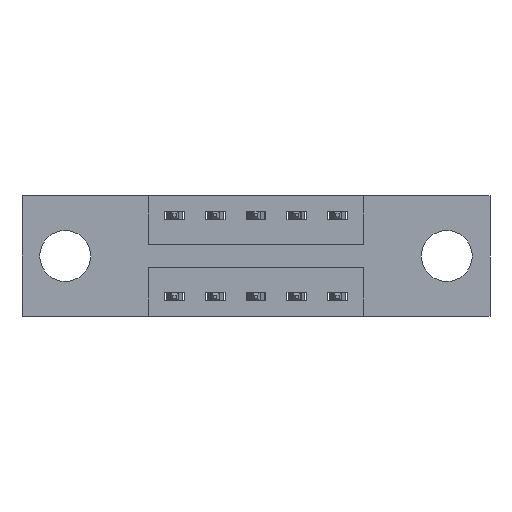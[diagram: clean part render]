
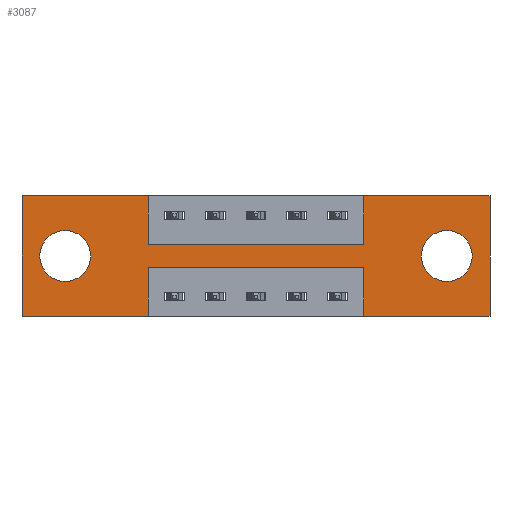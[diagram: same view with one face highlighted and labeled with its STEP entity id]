
A CAD part, front view. The second image highlights one B-rep face of the part: STEP entity #3087.
In plain terms, the highlighted planar face has unit normal (0, -1, 0).
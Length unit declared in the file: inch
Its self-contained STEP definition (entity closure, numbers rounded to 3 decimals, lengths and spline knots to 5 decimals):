
#97 = CARTESIAN_POINT ( 'NONE',  ( 0.3875, 0., -0.15 ) ) ;
#135 = CARTESIAN_POINT ( 'NONE',  ( 1.435, 0., 0. ) ) ;
#159 = ORIENTED_EDGE ( 'NONE', *, *, #3614, .F. ) ;
#218 = CARTESIAN_POINT ( 'NONE',  ( 0., 0., -0.37 ) ) ;
#339 = DIRECTION ( 'NONE',  ( 0., 0., 1. ) ) ;
#363 = ORIENTED_EDGE ( 'NONE', *, *, #2648, .F. ) ;
#393 = FACE_BOUND ( 'NONE', #5636, .T. ) ;
#713 = VERTEX_POINT ( 'NONE', #7406 ) ;
#732 = ORIENTED_EDGE ( 'NONE', *, *, #6379, .F. ) ;
#763 = CARTESIAN_POINT ( 'NONE',  ( 0., 0., -0.37 ) ) ;
#812 = EDGE_CURVE ( 'NONE', #1909, #713, #1612, .T. ) ;
#863 = CARTESIAN_POINT ( 'NONE',  ( 1.0475, 0., -0.37 ) ) ;
#921 = FACE_OUTER_BOUND ( 'NONE', #5794, .T. ) ;
#931 = EDGE_CURVE ( 'NONE', #5371, #4724, #8557, .T. ) ;
#1012 = CARTESIAN_POINT ( 'NONE',  ( 1.435, 0., 0. ) ) ;
#1031 = LINE ( 'NONE', #3016, #7237 ) ;
#1059 = CARTESIAN_POINT ( 'NONE',  ( 0.3875, 0., -0.15 ) ) ;
#1108 = DIRECTION ( 'NONE',  ( 0., 0., -1. ) ) ;
#1122 = VERTEX_POINT ( 'NONE', #97 ) ;
#1137 = ORIENTED_EDGE ( 'NONE', *, *, #4799, .F. ) ;
#1143 = CARTESIAN_POINT ( 'NONE',  ( 0.3875, 0., 0. ) ) ;
#1146 = VERTEX_POINT ( 'NONE', #4789 ) ;
#1202 = AXIS2_PLACEMENT_3D ( 'NONE', #7115, #8446, #1108 ) ;
#1241 = DIRECTION ( 'NONE',  ( 1., 0., 0. ) ) ;
#1268 = CARTESIAN_POINT ( 'NONE',  ( 0.3875, 0., 0. ) ) ;
#1274 = CARTESIAN_POINT ( 'NONE',  ( 1.3025, 0., -0.185 ) ) ;
#1301 = ORIENTED_EDGE ( 'NONE', *, *, #7108, .F. ) ;
#1328 = LINE ( 'NONE', #4021, #6715 ) ;
#1489 = LINE ( 'NONE', #763, #7800 ) ;
#1612 = CIRCLE ( 'NONE', #6519, 0.078 ) ;
#1732 = DIRECTION ( 'NONE',  ( 0., -1., 0. ) ) ;
#1733 = VERTEX_POINT ( 'NONE', #3172 ) ;
#1747 = VECTOR ( 'NONE', #1241, 39.37008 ) ;
#1909 = VERTEX_POINT ( 'NONE', #2915 ) ;
#1947 = VERTEX_POINT ( 'NONE', #8504 ) ;
#1992 = CARTESIAN_POINT ( 'NONE',  ( 0.1325, 0., -0.185 ) ) ;
#2010 = DIRECTION ( 'NONE',  ( 0., 0., -1. ) ) ;
#2065 = ORIENTED_EDGE ( 'NONE', *, *, #812, .T. ) ;
#2088 = LINE ( 'NONE', #1012, #4462 ) ;
#2157 = ORIENTED_EDGE ( 'NONE', *, *, #3363, .T. ) ;
#2252 = CARTESIAN_POINT ( 'NONE',  ( 1.3025, 0., -0.263 ) ) ;
#2350 = VECTOR ( 'NONE', #6052, 39.37008 ) ;
#2438 = CARTESIAN_POINT ( 'NONE',  ( 0., 0., 0. ) ) ;
#2447 = CARTESIAN_POINT ( 'NONE',  ( 0., 0., -0.37 ) ) ;
#2479 = EDGE_CURVE ( 'NONE', #3506, #7381, #5400, .T. ) ;
#2648 = EDGE_CURVE ( 'NONE', #1733, #1947, #1489, .T. ) ;
#2780 = DIRECTION ( 'NONE',  ( 0., 1., 0. ) ) ;
#2801 = DIRECTION ( 'NONE',  ( 0., 1., 0. ) ) ;
#2915 = CARTESIAN_POINT ( 'NONE',  ( 0.1325, 0., -0.107 ) ) ;
#3013 = VERTEX_POINT ( 'NONE', #4783 ) ;
#3016 = CARTESIAN_POINT ( 'NONE',  ( 0., 0., 0. ) ) ;
#3087 = ADVANCED_FACE ( 'NONE', ( #393, #7660, #921 ), #3730, .T. ) ;
#3172 = CARTESIAN_POINT ( 'NONE',  ( 0.3875, 0., -0.37 ) ) ;
#3203 = CARTESIAN_POINT ( 'NONE',  ( 0., 0., 0. ) ) ;
#3319 = EDGE_CURVE ( 'NONE', #1947, #7468, #4738, .T. ) ;
#3356 = ORIENTED_EDGE ( 'NONE', *, *, #5023, .F. ) ;
#3363 = EDGE_CURVE ( 'NONE', #713, #1909, #6764, .T. ) ;
#3379 = LINE ( 'NONE', #8691, #2350 ) ;
#3506 = VERTEX_POINT ( 'NONE', #2252 ) ;
#3558 = CARTESIAN_POINT ( 'NONE',  ( 1.0475, 0., -0.15 ) ) ;
#3614 = EDGE_CURVE ( 'NONE', #1122, #7260, #4513, .T. ) ;
#3642 = ORIENTED_EDGE ( 'NONE', *, *, #4659, .F. ) ;
#3693 = DIRECTION ( 'NONE',  ( 1., 0., 0. ) ) ;
#3730 = PLANE ( 'NONE',  #8400 ) ;
#3757 = ORIENTED_EDGE ( 'NONE', *, *, #931, .F. ) ;
#3799 = ORIENTED_EDGE ( 'NONE', *, *, #3319, .F. ) ;
#4021 = CARTESIAN_POINT ( 'NONE',  ( 0.3875, 0., -0.22 ) ) ;
#4042 = EDGE_CURVE ( 'NONE', #6018, #1146, #7189, .T. ) ;
#4063 = DIRECTION ( 'NONE',  ( 0., 0., 1. ) ) ;
#4083 = DIRECTION ( 'NONE',  ( 0., 0., -1. ) ) ;
#4185 = EDGE_CURVE ( 'NONE', #8071, #1733, #5927, .T. ) ;
#4272 = AXIS2_PLACEMENT_3D ( 'NONE', #1992, #2780, #4063 ) ;
#4462 = VECTOR ( 'NONE', #7739, 39.37008 ) ;
#4472 = EDGE_CURVE ( 'NONE', #7468, #8417, #1031, .T. ) ;
#4513 = LINE ( 'NONE', #1059, #1747 ) ;
#4659 = EDGE_CURVE ( 'NONE', #7260, #5371, #3379, .T. ) ;
#4721 = VECTOR ( 'NONE', #3693, 39.37008 ) ;
#4724 = VERTEX_POINT ( 'NONE', #135 ) ;
#4738 = LINE ( 'NONE', #6720, #7328 ) ;
#4783 = CARTESIAN_POINT ( 'NONE',  ( 1.0475, 0., -0.22 ) ) ;
#4789 = CARTESIAN_POINT ( 'NONE',  ( 1.0475, 0., -0.37 ) ) ;
#4799 = EDGE_CURVE ( 'NONE', #4724, #6018, #2088, .T. ) ;
#4869 = DIRECTION ( 'NONE',  ( 0., 0., 1. ) ) ;
#4911 = LINE ( 'NONE', #863, #6435 ) ;
#5023 = EDGE_CURVE ( 'NONE', #3013, #8071, #1328, .T. ) ;
#5209 = ORIENTED_EDGE ( 'NONE', *, *, #4185, .F. ) ;
#5211 = CARTESIAN_POINT ( 'NONE',  ( 0.3875, 0., -0.22 ) ) ;
#5268 = CARTESIAN_POINT ( 'NONE',  ( 0.3875, 0., -0.37 ) ) ;
#5349 = LINE ( 'NONE', #1268, #5567 ) ;
#5371 = VERTEX_POINT ( 'NONE', #6447 ) ;
#5376 = ORIENTED_EDGE ( 'NONE', *, *, #2479, .T. ) ;
#5400 = CIRCLE ( 'NONE', #1202, 0.078 ) ;
#5445 = EDGE_CURVE ( 'NONE', #7381, #3506, #5774, .T. ) ;
#5477 = DIRECTION ( 'NONE',  ( 0., 0., 1. ) ) ;
#5567 = VECTOR ( 'NONE', #4083, 39.37008 ) ;
#5636 = EDGE_LOOP ( 'NONE', ( #7654, #5376 ) ) ;
#5774 = CIRCLE ( 'NONE', #6881, 0.078 ) ;
#5794 = EDGE_LOOP ( 'NONE', ( #5209, #3356, #732, #8390, #1137, #3757, #3642, #159, #1301, #8591, #3799, #363 ) ) ;
#5927 = LINE ( 'NONE', #5268, #8226 ) ;
#6018 = VERTEX_POINT ( 'NONE', #8547 ) ;
#6052 = DIRECTION ( 'NONE',  ( 0., 0., 1. ) ) ;
#6141 = DIRECTION ( 'NONE',  ( 0., 1., 0. ) ) ;
#6211 = EDGE_LOOP ( 'NONE', ( #2065, #2157 ) ) ;
#6270 = CARTESIAN_POINT ( 'NONE',  ( 0.1325, 0., -0.185 ) ) ;
#6379 = EDGE_CURVE ( 'NONE', #1146, #3013, #4911, .T. ) ;
#6435 = VECTOR ( 'NONE', #339, 39.37008 ) ;
#6447 = CARTESIAN_POINT ( 'NONE',  ( 1.0475, 0., 0. ) ) ;
#6484 = DIRECTION ( 'NONE',  ( -1., 0., 0. ) ) ;
#6519 = AXIS2_PLACEMENT_3D ( 'NONE', #6270, #6141, #5477 ) ;
#6526 = DIRECTION ( 'NONE',  ( 1., 0., 0. ) ) ;
#6715 = VECTOR ( 'NONE', #6797, 39.37008 ) ;
#6720 = CARTESIAN_POINT ( 'NONE',  ( 0., 0., 0. ) ) ;
#6764 = CIRCLE ( 'NONE', #4272, 0.078 ) ;
#6797 = DIRECTION ( 'NONE',  ( -1., 0., 0. ) ) ;
#6881 = AXIS2_PLACEMENT_3D ( 'NONE', #1274, #2801, #7409 ) ;
#6976 = DIRECTION ( 'NONE',  ( -1., 0., 0. ) ) ;
#7041 = DIRECTION ( 'NONE',  ( 0., 0., -1. ) ) ;
#7108 = EDGE_CURVE ( 'NONE', #8417, #1122, #5349, .T. ) ;
#7115 = CARTESIAN_POINT ( 'NONE',  ( 1.3025, 0., -0.185 ) ) ;
#7189 = LINE ( 'NONE', #2447, #7320 ) ;
#7237 = VECTOR ( 'NONE', #6526, 39.37008 ) ;
#7260 = VERTEX_POINT ( 'NONE', #3558 ) ;
#7320 = VECTOR ( 'NONE', #6484, 39.37008 ) ;
#7328 = VECTOR ( 'NONE', #4869, 39.37008 ) ;
#7381 = VERTEX_POINT ( 'NONE', #7840 ) ;
#7406 = CARTESIAN_POINT ( 'NONE',  ( 0.1325, 0., -0.263 ) ) ;
#7409 = DIRECTION ( 'NONE',  ( 0., 0., -1. ) ) ;
#7468 = VERTEX_POINT ( 'NONE', #2438 ) ;
#7654 = ORIENTED_EDGE ( 'NONE', *, *, #5445, .T. ) ;
#7660 = FACE_BOUND ( 'NONE', #6211, .T. ) ;
#7739 = DIRECTION ( 'NONE',  ( 0., 0., -1. ) ) ;
#7800 = VECTOR ( 'NONE', #6976, 39.37008 ) ;
#7840 = CARTESIAN_POINT ( 'NONE',  ( 1.3025, 0., -0.107 ) ) ;
#8071 = VERTEX_POINT ( 'NONE', #5211 ) ;
#8226 = VECTOR ( 'NONE', #2010, 39.37008 ) ;
#8390 = ORIENTED_EDGE ( 'NONE', *, *, #4042, .F. ) ;
#8400 = AXIS2_PLACEMENT_3D ( 'NONE', #218, #1732, #7041 ) ;
#8417 = VERTEX_POINT ( 'NONE', #1143 ) ;
#8446 = DIRECTION ( 'NONE',  ( 0., 1., 0. ) ) ;
#8504 = CARTESIAN_POINT ( 'NONE',  ( 0., 0., -0.37 ) ) ;
#8547 = CARTESIAN_POINT ( 'NONE',  ( 1.435, 0., -0.37 ) ) ;
#8557 = LINE ( 'NONE', #3203, #4721 ) ;
#8591 = ORIENTED_EDGE ( 'NONE', *, *, #4472, .F. ) ;
#8691 = CARTESIAN_POINT ( 'NONE',  ( 1.0475, 0., 0. ) ) ;
